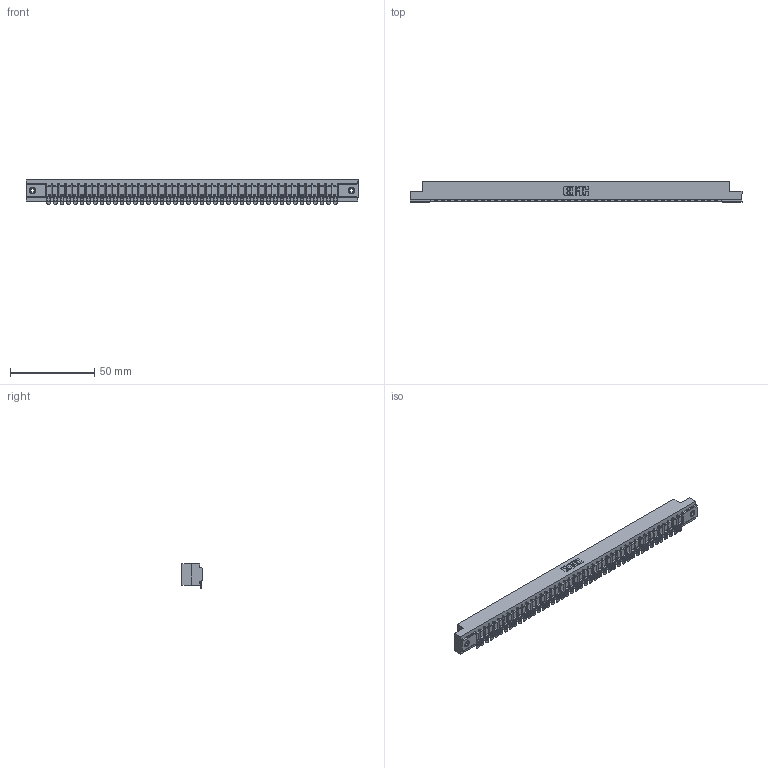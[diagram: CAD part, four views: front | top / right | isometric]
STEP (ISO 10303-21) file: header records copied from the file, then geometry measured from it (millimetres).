
FILE_DESCRIPTION (( 'STEP AP203' ), '1' );
FILE_NAME ('307-044-454-108.STEP', '2020-09-29T23:17:00', ( '' ), ( '' ), 'SwSTEP 2.0', 'SolidWorks 2020', '' );
FILE_SCHEMA (( 'CONFIG_CONTROL_DESIGN' ));
Length unit declared in the file: inch
Products named in the file (4): 307 Part_.156 Dia Mounting Holes; 345-250-001_345-250-003-102; 307-290-002_554; 307-044-454-108
Assembly tree (47 placements, depth 2):
  307-044-454-108
    307 Part_.156 Dia Mounting Holes
    307-290-002_554  x44
    345-250-001_345-250-003-102  x2
Bounding box: 197.36 x 12.01 x 14.52 mm (x, y, z)
Volume: 21144.1 mm3; surface area: 26818.4 mm2
Topology: 47 solids, 47 shells, 3787 faces, 11591 edges, 7598 vertices
Faces by surface type: plane 2126, cylinder 1555, sphere 90, cone 12, torus 4
Entity records: 39624 total; most frequent: CARTESIAN_POINT 6665, ORIENTED_EDGE 6648, DIRECTION 6490, EDGE_CURVE 3324, VECTOR 2540, LINE 2540, VERTEX_POINT 2150, AXIS2_PLACEMENT_3D 1975
